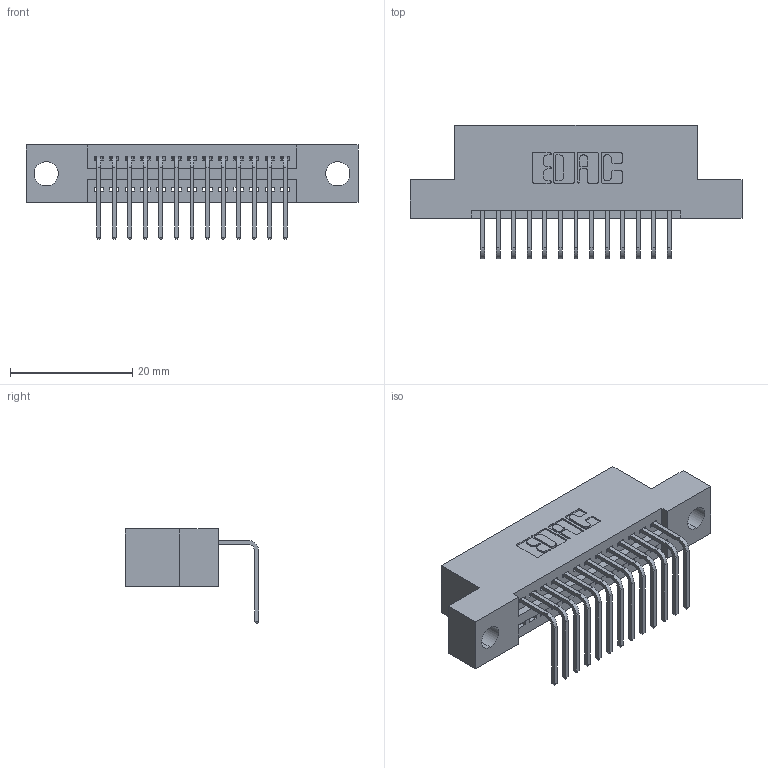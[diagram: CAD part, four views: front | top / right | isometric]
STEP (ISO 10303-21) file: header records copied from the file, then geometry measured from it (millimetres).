
FILE_DESCRIPTION (( 'STEP AP203' ), '1' );
FILE_NAME ('345-013-558-104.STEP', '2021-06-01T16:15:39', ( '' ), ( '' ), 'SwSTEP 2.0', 'SolidWorks 2020', '' );
FILE_SCHEMA (( 'CONFIG_CONTROL_DESIGN' ));
Length unit declared in the file: inch
Products named in the file (3): 345-292-001_558 Tail - 2; 345-013-558-104; 345 Part_Flush Mounting Lugs - 0.156 Dia-TI
Assembly tree (14 placements, depth 2):
  345-013-558-104
    345 Part_Flush Mounting Lugs - 0.156 Dia-TI
    345-292-001_558 Tail - 2  x13
Bounding box: 54.23 x 21.83 x 15.37 mm (x, y, z)
Volume: 4850.5 mm3; surface area: 6148.8 mm2
Topology: 14 solids, 14 shells, 920 faces, 2743 edges, 1810 vertices
Faces by surface type: plane 640, cylinder 280
Entity records: 14191 total; most frequent: CARTESIAN_POINT 2469, ORIENTED_EDGE 2414, DIRECTION 2197, EDGE_CURVE 1207, VECTOR 1023, LINE 1023, VERTEX_POINT 802, AXIS2_PLACEMENT_3D 587
